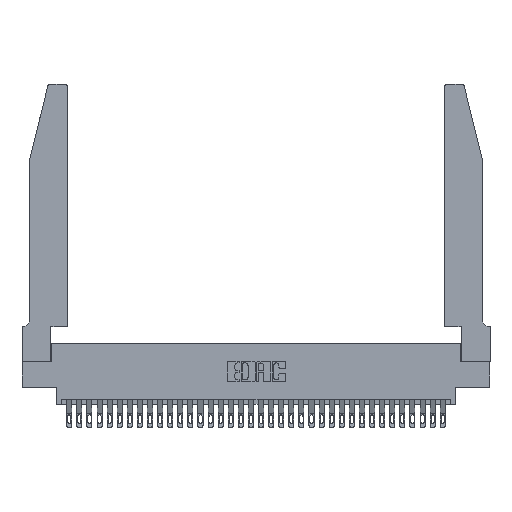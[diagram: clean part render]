
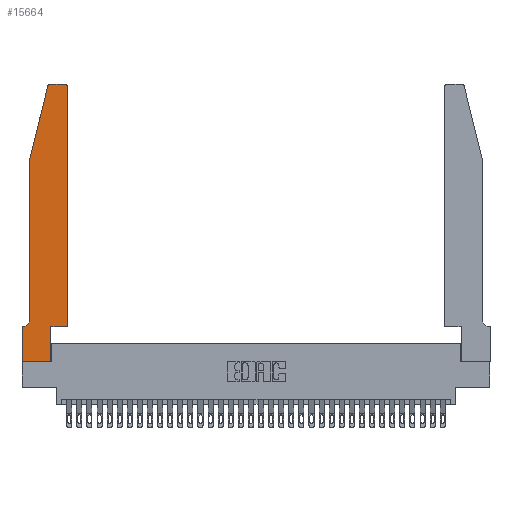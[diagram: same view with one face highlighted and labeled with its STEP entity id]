
A CAD part, top view. The second image highlights one B-rep face of the part: STEP entity #15664.
In plain terms, the highlighted planar face has unit normal (0, 0, 1).
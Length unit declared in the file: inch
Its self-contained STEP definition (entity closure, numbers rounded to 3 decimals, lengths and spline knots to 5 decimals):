
#436 = CARTESIAN_POINT ( 'NONE',  ( 0., 0.35, 0.37 ) ) ;
#892 = VECTOR ( 'NONE', #14456, 39.37008 ) ;
#1236 = CARTESIAN_POINT ( 'NONE',  ( 0.4505, 0.35, 0.37 ) ) ;
#1988 = LINE ( 'NONE', #9198, #25491 ) ;
#2117 = DIRECTION ( 'NONE',  ( 0., 0., 1. ) ) ;
#2686 = ORIENTED_EDGE ( 'NONE', *, *, #15263, .T. ) ;
#2893 = ORIENTED_EDGE ( 'NONE', *, *, #5192, .T. ) ;
#3055 = DIRECTION ( 'NONE',  ( -0.239, -0.971, 0. ) ) ;
#3102 = CARTESIAN_POINT ( 'NONE',  ( 0.2865, 0., 0.37 ) ) ;
#3257 = ORIENTED_EDGE ( 'NONE', *, *, #26850, .T. ) ;
#3739 = VERTEX_POINT ( 'NONE', #21480 ) ;
#4172 = EDGE_CURVE ( 'NONE', #3739, #25226, #31096, .T. ) ;
#4627 = ORIENTED_EDGE ( 'NONE', *, *, #10082, .T. ) ;
#4894 = VERTEX_POINT ( 'NONE', #18914 ) ;
#4903 = EDGE_CURVE ( 'NONE', #4894, #18220, #20316, .T. ) ;
#5063 = CIRCLE ( 'NONE', #16404, 0.03 ) ;
#5183 = VERTEX_POINT ( 'NONE', #30695 ) ;
#5192 = EDGE_CURVE ( 'NONE', #15172, #5183, #11205, .T. ) ;
#5746 = ORIENTED_EDGE ( 'NONE', *, *, #18534, .T. ) ;
#5756 = VECTOR ( 'NONE', #9139, 39.37008 ) ;
#5902 = CARTESIAN_POINT ( 'NONE',  ( 0.284, 2.72, 0.37 ) ) ;
#6022 = CARTESIAN_POINT ( 'NONE',  ( 0.25487, 2.72718, 0.37 ) ) ;
#6356 = DIRECTION ( 'NONE',  ( 1., 0., 0. ) ) ;
#6413 = CIRCLE ( 'NONE', #8794, 0.03 ) ;
#6427 = DIRECTION ( 'NONE',  ( 1., 0., 0. ) ) ;
#6680 = CARTESIAN_POINT ( 'NONE',  ( 0., 0.35, 0.37 ) ) ;
#6789 = DIRECTION ( 'NONE',  ( 0., 0., 1. ) ) ;
#6837 = CARTESIAN_POINT ( 'NONE',  ( 0.0755, 0.35, 0.37 ) ) ;
#7061 = AXIS2_PLACEMENT_3D ( 'NONE', #31165, #12047, #20480 ) ;
#7620 = CARTESIAN_POINT ( 'NONE',  ( 0.4505, 0.35, 0.37 ) ) ;
#7666 = CARTESIAN_POINT ( 'NONE',  ( 0.2865, 0.35, 0.37 ) ) ;
#7934 = DIRECTION ( 'NONE',  ( -1., 0., 0. ) ) ;
#8395 = LINE ( 'NONE', #1236, #19138 ) ;
#8450 = ORIENTED_EDGE ( 'NONE', *, *, #15042, .T. ) ;
#8482 = ORIENTED_EDGE ( 'NONE', *, *, #20810, .T. ) ;
#8594 = DIRECTION ( 'NONE',  ( 0., 0., 1. ) ) ;
#8794 = AXIS2_PLACEMENT_3D ( 'NONE', #5902, #8594, #6356 ) ;
#9139 = DIRECTION ( 'NONE',  ( 0., 1., 0. ) ) ;
#9198 = CARTESIAN_POINT ( 'NONE',  ( 0.4505, 0.35, 0.37 ) ) ;
#9435 = LINE ( 'NONE', #23008, #892 ) ;
#10082 = EDGE_CURVE ( 'NONE', #28746, #25423, #8395, .T. ) ;
#10277 = DIRECTION ( 'NONE',  ( -1., 0., 0. ) ) ;
#10278 = CARTESIAN_POINT ( 'NONE',  ( 0.0755, 0.42, 0.37 ) ) ;
#10854 = VERTEX_POINT ( 'NONE', #10278 ) ;
#10883 = CARTESIAN_POINT ( 'NONE',  ( 0., 0., 0.37 ) ) ;
#11205 = LINE ( 'NONE', #16888, #30579 ) ;
#11588 = DIRECTION ( 'NONE',  ( 1., 0., 0. ) ) ;
#12034 = EDGE_LOOP ( 'NONE', ( #20001, #5746, #2893, #8450, #8482, #19966, #27010, #34928, #19699, #4627, #2686, #3257 ) ) ;
#12047 = DIRECTION ( 'NONE',  ( 0., 0., -1. ) ) ;
#12996 = LINE ( 'NONE', #35437, #33202 ) ;
#13074 = CARTESIAN_POINT ( 'NONE',  ( 0.4205, 2.72, 0.37 ) ) ;
#14007 = CARTESIAN_POINT ( 'NONE',  ( 0.4505, 2.72, 0.37 ) ) ;
#14456 = DIRECTION ( 'NONE',  ( 1., 0., 0. ) ) ;
#14623 = DIRECTION ( 'NONE',  ( 0., -1., 0. ) ) ;
#15042 = EDGE_CURVE ( 'NONE', #5183, #10854, #17777, .T. ) ;
#15172 = VERTEX_POINT ( 'NONE', #6022 ) ;
#15263 = EDGE_CURVE ( 'NONE', #25423, #25073, #1988, .T. ) ;
#15664 = ADVANCED_FACE ( 'NONE', ( #23736 ), #17333, .T. ) ;
#15706 = EDGE_CURVE ( 'NONE', #15856, #28746, #18600, .T. ) ;
#15856 = VERTEX_POINT ( 'NONE', #3102 ) ;
#16404 = AXIS2_PLACEMENT_3D ( 'NONE', #13074, #2117, #21276 ) ;
#16716 = EDGE_CURVE ( 'NONE', #18220, #23248, #12996, .T. ) ;
#16888 = CARTESIAN_POINT ( 'NONE',  ( 0.0755, 2., 0.37 ) ) ;
#17333 = PLANE ( 'NONE',  #30411 ) ;
#17777 = LINE ( 'NONE', #20030, #35047 ) ;
#17966 = EDGE_CURVE ( 'NONE', #23248, #15856, #9435, .T. ) ;
#18220 = VERTEX_POINT ( 'NONE', #6680 ) ;
#18534 = EDGE_CURVE ( 'NONE', #25226, #15172, #6413, .T. ) ;
#18600 = LINE ( 'NONE', #19960, #5756 ) ;
#18914 = CARTESIAN_POINT ( 'NONE',  ( 0.0055, 0.35, 0.37 ) ) ;
#19138 = VECTOR ( 'NONE', #11588, 39.37008 ) ;
#19699 = ORIENTED_EDGE ( 'NONE', *, *, #15706, .T. ) ;
#19960 = CARTESIAN_POINT ( 'NONE',  ( 0.2865, 0.35, 0.37 ) ) ;
#19966 = ORIENTED_EDGE ( 'NONE', *, *, #4903, .T. ) ;
#20001 = ORIENTED_EDGE ( 'NONE', *, *, #4172, .T. ) ;
#20030 = CARTESIAN_POINT ( 'NONE',  ( 0.0755, 2., 0.37 ) ) ;
#20156 = DIRECTION ( 'NONE',  ( 0., 1., 0. ) ) ;
#20316 = LINE ( 'NONE', #6837, #21639 ) ;
#20480 = DIRECTION ( 'NONE',  ( -1., 0., 0. ) ) ;
#20810 = EDGE_CURVE ( 'NONE', #10854, #4894, #29808, .T. ) ;
#21276 = DIRECTION ( 'NONE',  ( 1., 0., 0. ) ) ;
#21480 = CARTESIAN_POINT ( 'NONE',  ( 0.4205, 2.75, 0.37 ) ) ;
#21639 = VECTOR ( 'NONE', #10277, 39.37008 ) ;
#22119 = VECTOR ( 'NONE', #7934, 39.37008 ) ;
#23008 = CARTESIAN_POINT ( 'NONE',  ( 0., 0., 0.37 ) ) ;
#23248 = VERTEX_POINT ( 'NONE', #10883 ) ;
#23736 = FACE_OUTER_BOUND ( 'NONE', #12034, .T. ) ;
#24509 = CARTESIAN_POINT ( 'NONE',  ( 0.2605, 2.75, 0.37 ) ) ;
#25073 = VERTEX_POINT ( 'NONE', #14007 ) ;
#25226 = VERTEX_POINT ( 'NONE', #28366 ) ;
#25423 = VERTEX_POINT ( 'NONE', #7620 ) ;
#25491 = VECTOR ( 'NONE', #20156, 39.37008 ) ;
#26850 = EDGE_CURVE ( 'NONE', #25073, #3739, #5063, .T. ) ;
#27010 = ORIENTED_EDGE ( 'NONE', *, *, #16716, .T. ) ;
#27174 = DIRECTION ( 'NONE',  ( 0., -1., 0. ) ) ;
#28366 = CARTESIAN_POINT ( 'NONE',  ( 0.284, 2.75, 0.37 ) ) ;
#28746 = VERTEX_POINT ( 'NONE', #7666 ) ;
#29808 = CIRCLE ( 'NONE', #7061, 0.07 ) ;
#30411 = AXIS2_PLACEMENT_3D ( 'NONE', #436, #6789, #6427 ) ;
#30579 = VECTOR ( 'NONE', #3055, 39.37008 ) ;
#30695 = CARTESIAN_POINT ( 'NONE',  ( 0.0755, 2., 0.37 ) ) ;
#31096 = LINE ( 'NONE', #24509, #22119 ) ;
#31165 = CARTESIAN_POINT ( 'NONE',  ( 0.0055, 0.42, 0.37 ) ) ;
#33202 = VECTOR ( 'NONE', #27174, 39.37008 ) ;
#34928 = ORIENTED_EDGE ( 'NONE', *, *, #17966, .T. ) ;
#35047 = VECTOR ( 'NONE', #14623, 39.37008 ) ;
#35437 = CARTESIAN_POINT ( 'NONE',  ( 0., 0., 0.37 ) ) ;
